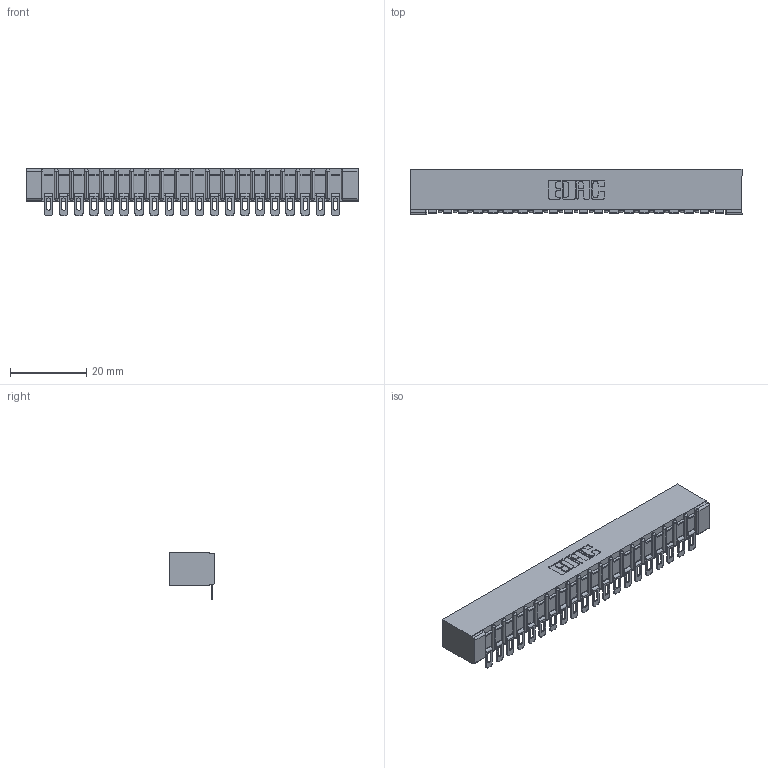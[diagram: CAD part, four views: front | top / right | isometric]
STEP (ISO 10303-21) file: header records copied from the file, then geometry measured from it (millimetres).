
FILE_DESCRIPTION (( 'STEP AP203' ), '1' );
FILE_NAME ('307-020-554-101.STEP', '2018-08-04T01:19:34', ( '' ), ( '' ), 'SwSTEP 2.0', 'SolidWorks 2016', '' );
FILE_SCHEMA (( 'CONFIG_CONTROL_DESIGN' ));
Length unit declared in the file: inch
Products named in the file (3): 307 Part_No Mounting Lugs; 307-290-002_554; 307-020-554-101
Assembly tree (21 placements, depth 2):
  307-020-554-101
    307 Part_No Mounting Lugs
    307-290-002_554  x20
Bounding box: 87.12 x 12.01 x 12.52 mm (x, y, z)
Volume: 6000.1 mm3; surface area: 11391.5 mm2
Topology: 21 solids, 21 shells, 1751 faces, 5359 edges, 3514 vertices
Faces by surface type: plane 986, cylinder 723, sphere 42
Entity records: 20545 total; most frequent: CARTESIAN_POINT 3462, ORIENTED_EDGE 3452, DIRECTION 3378, EDGE_CURVE 1726, VECTOR 1306, LINE 1306, VERTEX_POINT 1120, AXIS2_PLACEMENT_3D 1036
